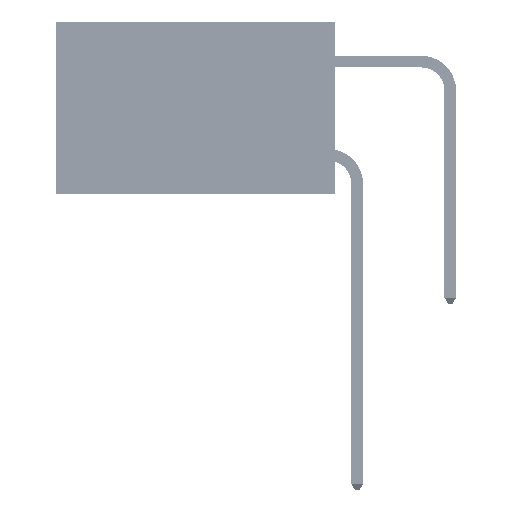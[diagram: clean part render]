
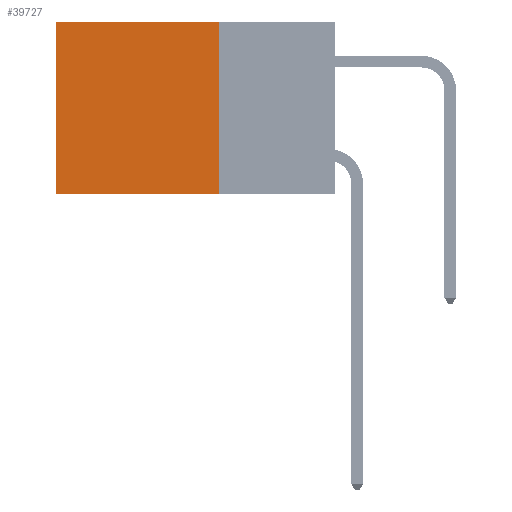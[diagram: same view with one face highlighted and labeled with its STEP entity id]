
A CAD part, left-side view. The second image highlights one B-rep face of the part: STEP entity #39727.
In plain terms, the highlighted planar face has unit normal (-1, 0, 0).
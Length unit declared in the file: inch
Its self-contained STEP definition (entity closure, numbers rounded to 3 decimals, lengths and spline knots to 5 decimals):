
#155 = EDGE_CURVE ( 'NONE', #42702, #15384, #53946, .T. ) ;
#894 = VECTOR ( 'NONE', #20789, 39.37008 ) ;
#4565 = EDGE_CURVE ( 'NONE', #31323, #52814, #35921, .T. ) ;
#6984 = AXIS2_PLACEMENT_3D ( 'NONE', #9603, #13870, #21817 ) ;
#8983 = DIRECTION ( 'NONE',  ( 0., 1., 0. ) ) ;
#9603 = CARTESIAN_POINT ( 'NONE',  ( 0.2875, 0.25, 0. ) ) ;
#11656 = CARTESIAN_POINT ( 'NONE',  ( 0.2875, 0.6, -0.37 ) ) ;
#12482 = LINE ( 'NONE', #47008, #35614 ) ;
#13376 = EDGE_CURVE ( 'NONE', #52814, #15384, #12482, .T. ) ;
#13870 = DIRECTION ( 'NONE',  ( 1., 0., 0. ) ) ;
#14163 = ORIENTED_EDGE ( 'NONE', *, *, #4565, .F. ) ;
#15260 = FACE_OUTER_BOUND ( 'NONE', #23472, .T. ) ;
#15384 = VERTEX_POINT ( 'NONE', #11656 ) ;
#16930 = DIRECTION ( 'NONE',  ( 0., 1., 0. ) ) ;
#17303 = ORIENTED_EDGE ( 'NONE', *, *, #39173, .T. ) ;
#17325 = VECTOR ( 'NONE', #8983, 39.37008 ) ;
#17766 = CARTESIAN_POINT ( 'NONE',  ( 0.2875, 0.6, 0. ) ) ;
#20789 = DIRECTION ( 'NONE',  ( 0., 0., -1. ) ) ;
#20947 = VECTOR ( 'NONE', #21656, 39.37008 ) ;
#21656 = DIRECTION ( 'NONE',  ( 0., 0., -1. ) ) ;
#21817 = DIRECTION ( 'NONE',  ( 0., 0., -1. ) ) ;
#23472 = EDGE_LOOP ( 'NONE', ( #47418, #23679, #14163, #17303 ) ) ;
#23679 = ORIENTED_EDGE ( 'NONE', *, *, #13376, .F. ) ;
#23963 = LINE ( 'NONE', #42605, #17325 ) ;
#30286 = CARTESIAN_POINT ( 'NONE',  ( 0.2875, 0.25, 0. ) ) ;
#31323 = VERTEX_POINT ( 'NONE', #30286 ) ;
#34891 = PLANE ( 'NONE',  #6984 ) ;
#35050 = CARTESIAN_POINT ( 'NONE',  ( 0.2875, 0.6, 0. ) ) ;
#35614 = VECTOR ( 'NONE', #16930, 39.37008 ) ;
#35921 = LINE ( 'NONE', #54329, #894 ) ;
#39173 = EDGE_CURVE ( 'NONE', #31323, #42702, #23963, .T. ) ;
#39727 = ADVANCED_FACE ( 'NONE', ( #15260 ), #34891, .F. ) ;
#41053 = CARTESIAN_POINT ( 'NONE',  ( 0.2875, 0.25, -0.37 ) ) ;
#42605 = CARTESIAN_POINT ( 'NONE',  ( 0.2875, 0.25, 0. ) ) ;
#42702 = VERTEX_POINT ( 'NONE', #35050 ) ;
#47008 = CARTESIAN_POINT ( 'NONE',  ( 0.2875, 0.25, -0.37 ) ) ;
#47418 = ORIENTED_EDGE ( 'NONE', *, *, #155, .T. ) ;
#52814 = VERTEX_POINT ( 'NONE', #41053 ) ;
#53946 = LINE ( 'NONE', #17766, #20947 ) ;
#54329 = CARTESIAN_POINT ( 'NONE',  ( 0.2875, 0.25, 0. ) ) ;
